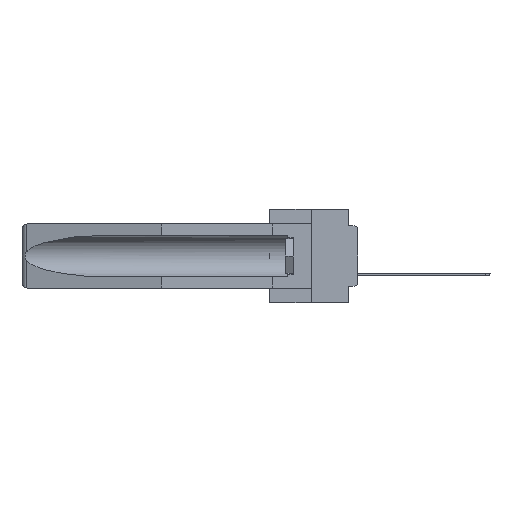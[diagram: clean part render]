
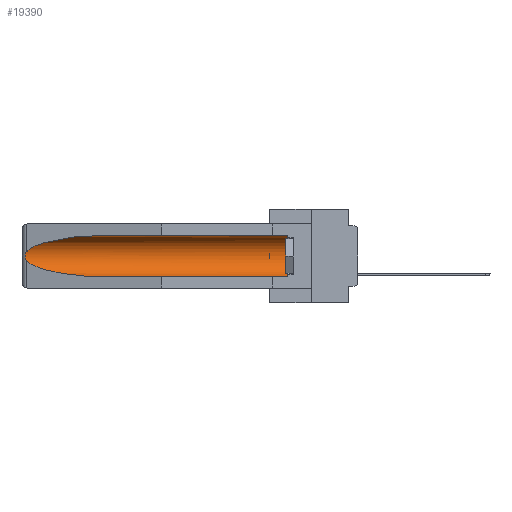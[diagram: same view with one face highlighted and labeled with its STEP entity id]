
A CAD part, left-side view. The second image highlights one B-rep face of the part: STEP entity #19390.
In plain terms, the highlighted cylindrical face has radius 2.857 mm (diameter 5.715 mm), a partial arc.
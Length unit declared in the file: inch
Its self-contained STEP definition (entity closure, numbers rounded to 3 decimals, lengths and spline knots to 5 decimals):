
#329 = EDGE_CURVE ( 'NONE', #14238, #22272, #30385, .T. ) ;
#2102 = DIRECTION ( 'NONE',  ( 0., 1., 0. ) ) ;
#2747 = VERTEX_POINT ( 'NONE', #29554 ) ;
#3401 = ORIENTED_EDGE ( 'NONE', *, *, #5966, .T. ) ;
#3740 = CARTESIAN_POINT ( 'NONE',  ( 0.26537, 1.52718, -0.14972 ) ) ;
#4241 = CARTESIAN_POINT ( 'NONE',  ( 0.25451, 1.48313, -0.24835 ) ) ;
#5966 = EDGE_CURVE ( 'NONE', #22272, #24073, #19144, .T. ) ;
#6330 =( BOUNDED_CURVE ( )  B_SPLINE_CURVE ( 3, ( #32625, #15279, #12243, #30407 ),
 .UNSPECIFIED., .F., .T. ) 
 B_SPLINE_CURVE_WITH_KNOTS ( ( 4, 4 ),
 ( 4.71239, 6.08839 ),
 .UNSPECIFIED. ) 
 CURVE ( )  GEOMETRIC_REPRESENTATION_ITEM ( )  RATIONAL_B_SPLINE_CURVE ( ( 1., 0.848, 0.848, 1. ) ) 
 REPRESENTATION_ITEM ( '' )  );
#6843 = DIRECTION ( 'NONE',  ( 0., 1., 0. ) ) ;
#7459 = ORIENTED_EDGE ( 'NONE', *, *, #18174, .F. ) ;
#8450 = AXIS2_PLACEMENT_3D ( 'NONE', #32361, #11195, #13606 ) ;
#8563 = LINE ( 'NONE', #38837, #38179 ) ;
#9395 = CARTESIAN_POINT ( 'NONE',  ( 0.26537, 1.52718, -0.19328 ) ) ;
#9880 = EDGE_CURVE ( 'NONE', #11922, #2747, #16573, .T. ) ;
#10824 = DIRECTION ( 'NONE',  ( 0., 1., 0. ) ) ;
#10931 = EDGE_CURVE ( 'NONE', #2747, #36580, #17397, .T. ) ;
#11195 = DIRECTION ( 'NONE',  ( 0., -1., 0. ) ) ;
#11922 = VERTEX_POINT ( 'NONE', #17784 ) ;
#12243 = CARTESIAN_POINT ( 'NONE',  ( 0.25451, 1.48313, -0.09465 ) ) ;
#13014 = CARTESIAN_POINT ( 'NONE',  ( 0.26654, 1.53092, -0.15636 ) ) ;
#13606 = DIRECTION ( 'NONE',  ( 0., 0., 1. ) ) ;
#14143 = ORIENTED_EDGE ( 'NONE', *, *, #9880, .T. ) ;
#14238 = VERTEX_POINT ( 'NONE', #34130 ) ;
#15279 = CARTESIAN_POINT ( 'NONE',  ( 0.21114, 1.30732, -0.059 ) ) ;
#15845 = CARTESIAN_POINT ( 'NONE',  ( 0.26597, 1.52961, -0.15275 ) ) ;
#16573 = B_SPLINE_CURVE_WITH_KNOTS ( 'NONE', 3,
 ( #3740, #15845, #13014, #22277, #19451, #19065, #31766, #28331, #25298, #9395 ),
 .UNSPECIFIED., .F., .F.,
 ( 4, 2, 2, 2, 4 ),
 ( 0., 0.00029, 0.00058, 0.00087, 0.00117 ),
 .UNSPECIFIED. ) ;
#16663 = EDGE_CURVE ( 'NONE', #24073, #11922, #6330, .T. ) ;
#16849 = CARTESIAN_POINT ( 'NONE',  ( 0.155, -0.30754, -0.1715 ) ) ;
#17134 = CARTESIAN_POINT ( 'NONE',  ( 0.21114, 1.30732, -0.284 ) ) ;
#17397 =( BOUNDED_CURVE ( )  B_SPLINE_CURVE ( 3, ( #22780, #4241, #17134, #35476 ),
 .UNSPECIFIED., .F., .T. ) 
 B_SPLINE_CURVE_WITH_KNOTS ( ( 4, 4 ),
 ( 0.1948, 1.5708 ),
 .UNSPECIFIED. ) 
 CURVE ( )  GEOMETRIC_REPRESENTATION_ITEM ( )  RATIONAL_B_SPLINE_CURVE ( ( 1., 0.848, 0.848, 1. ) ) 
 REPRESENTATION_ITEM ( '' )  );
#17767 = ORIENTED_EDGE ( 'NONE', *, *, #329, .T. ) ;
#17784 = CARTESIAN_POINT ( 'NONE',  ( 0.26537, 1.52718, -0.14972 ) ) ;
#17903 = AXIS2_PLACEMENT_3D ( 'NONE', #16849, #10824, #23097 ) ;
#18174 = EDGE_CURVE ( 'NONE', #14238, #36580, #8563, .T. ) ;
#19065 = CARTESIAN_POINT ( 'NONE',  ( 0.2675, 1.53308, -0.17534 ) ) ;
#19144 = LINE ( 'NONE', #34476, #19425 ) ;
#19390 = ADVANCED_FACE ( 'NONE', ( #35609 ), #31999, .F. ) ;
#19425 = VECTOR ( 'NONE', #6843, 39.37008 ) ;
#19451 = CARTESIAN_POINT ( 'NONE',  ( 0.2675, 1.53308, -0.16763 ) ) ;
#22259 = CARTESIAN_POINT ( 'NONE',  ( 0.155, 1.07973, -0.059 ) ) ;
#22272 = VERTEX_POINT ( 'NONE', #25769 ) ;
#22277 = CARTESIAN_POINT ( 'NONE',  ( 0.2673, 1.5327, -0.16383 ) ) ;
#22613 = ORIENTED_EDGE ( 'NONE', *, *, #16663, .T. ) ;
#22780 = CARTESIAN_POINT ( 'NONE',  ( 0.26537, 1.52718, -0.19328 ) ) ;
#23097 = DIRECTION ( 'NONE',  ( 0., 0., 1. ) ) ;
#24073 = VERTEX_POINT ( 'NONE', #22259 ) ;
#25298 = CARTESIAN_POINT ( 'NONE',  ( 0.26597, 1.5296, -0.19026 ) ) ;
#25769 = CARTESIAN_POINT ( 'NONE',  ( 0.155, 0.126, -0.059 ) ) ;
#28331 = CARTESIAN_POINT ( 'NONE',  ( 0.26655, 1.53094, -0.18657 ) ) ;
#29402 = EDGE_LOOP ( 'NONE', ( #22613, #14143, #38675, #7459, #17767, #3401 ) ) ;
#29554 = CARTESIAN_POINT ( 'NONE',  ( 0.26537, 1.52718, -0.19328 ) ) ;
#30385 = CIRCLE ( 'NONE', #8450, 0.1125 ) ;
#30407 = CARTESIAN_POINT ( 'NONE',  ( 0.26537, 1.52718, -0.14972 ) ) ;
#31766 = CARTESIAN_POINT ( 'NONE',  ( 0.2673, 1.53269, -0.17917 ) ) ;
#31999 = CYLINDRICAL_SURFACE ( 'NONE', #17903, 0.1125 ) ;
#32361 = CARTESIAN_POINT ( 'NONE',  ( 0.155, 0.126, -0.1715 ) ) ;
#32625 = CARTESIAN_POINT ( 'NONE',  ( 0.155, 1.07973, -0.059 ) ) ;
#34130 = CARTESIAN_POINT ( 'NONE',  ( 0.155, 0.126, -0.284 ) ) ;
#34476 = CARTESIAN_POINT ( 'NONE',  ( 0.155, -0.30754, -0.059 ) ) ;
#35476 = CARTESIAN_POINT ( 'NONE',  ( 0.155, 1.07973, -0.284 ) ) ;
#35609 = FACE_OUTER_BOUND ( 'NONE', #29402, .T. ) ;
#36580 = VERTEX_POINT ( 'NONE', #36835 ) ;
#36835 = CARTESIAN_POINT ( 'NONE',  ( 0.155, 1.07973, -0.284 ) ) ;
#38179 = VECTOR ( 'NONE', #2102, 39.37008 ) ;
#38675 = ORIENTED_EDGE ( 'NONE', *, *, #10931, .T. ) ;
#38837 = CARTESIAN_POINT ( 'NONE',  ( 0.155, -0.30754, -0.284 ) ) ;
